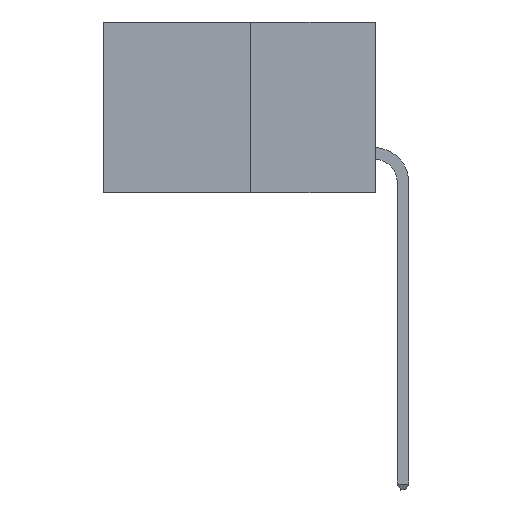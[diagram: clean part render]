
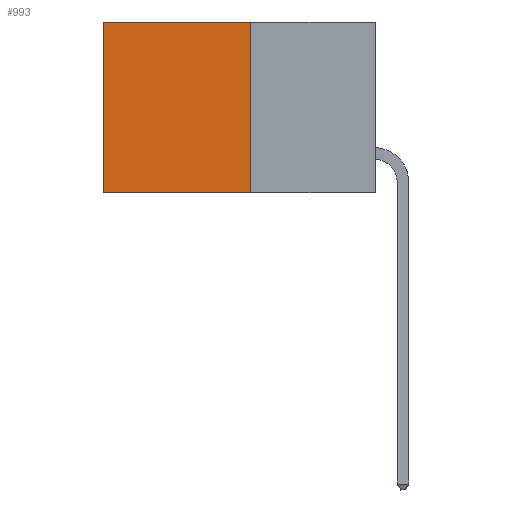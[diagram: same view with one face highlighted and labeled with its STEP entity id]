
A CAD part, left-side view. The second image highlights one B-rep face of the part: STEP entity #993.
In plain terms, the highlighted planar face has unit normal (-1, 0, 0).
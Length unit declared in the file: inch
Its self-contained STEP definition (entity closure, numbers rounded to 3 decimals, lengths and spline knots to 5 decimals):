
#87 = LINE ( 'NONE', #1131, #11337 ) ;
#577 = EDGE_CURVE ( 'NONE', #2310, #938, #10848, .T. ) ;
#585 = DIRECTION ( 'NONE',  ( 0., 1., 0. ) ) ;
#938 = VERTEX_POINT ( 'NONE', #11036 ) ;
#993 = ADVANCED_FACE ( 'NONE', ( #7029 ), #5491, .F. ) ;
#1131 = CARTESIAN_POINT ( 'NONE',  ( 0.277, 0.59, -0.37 ) ) ;
#1203 = DIRECTION ( 'NONE',  ( 0., 0., -1. ) ) ;
#1781 = VECTOR ( 'NONE', #585, 39.37008 ) ;
#2198 = VERTEX_POINT ( 'NONE', #9587 ) ;
#2310 = VERTEX_POINT ( 'NONE', #6604 ) ;
#2346 = EDGE_CURVE ( 'NONE', #10429, #2198, #8640, .T. ) ;
#3543 = VECTOR ( 'NONE', #5954, 39.37008 ) ;
#4050 = LINE ( 'NONE', #11639, #11327 ) ;
#4803 = CARTESIAN_POINT ( 'NONE',  ( 0.277, 0.27, -0.37 ) ) ;
#4816 = CARTESIAN_POINT ( 'NONE',  ( 0.277, 0.27, 0. ) ) ;
#5102 = ORIENTED_EDGE ( 'NONE', *, *, #10479, .T. ) ;
#5336 = DIRECTION ( 'NONE',  ( 0., 0., -1. ) ) ;
#5491 = PLANE ( 'NONE',  #8079 ) ;
#5525 = CARTESIAN_POINT ( 'NONE',  ( 0.277, 0.27, 0. ) ) ;
#5954 = DIRECTION ( 'NONE',  ( 0., 1., 0. ) ) ;
#5956 = EDGE_LOOP ( 'NONE', ( #5102, #6935, #9717, #8720 ) ) ;
#6604 = CARTESIAN_POINT ( 'NONE',  ( 0.277, 0.27, -0.37 ) ) ;
#6827 = DIRECTION ( 'NONE',  ( 0., 0., -1. ) ) ;
#6935 = ORIENTED_EDGE ( 'NONE', *, *, #577, .F. ) ;
#7029 = FACE_OUTER_BOUND ( 'NONE', #5956, .T. ) ;
#7379 = EDGE_CURVE ( 'NONE', #10429, #2310, #4050, .T. ) ;
#8079 = AXIS2_PLACEMENT_3D ( 'NONE', #4803, #8428, #1203 ) ;
#8428 = DIRECTION ( 'NONE',  ( 1., 0., 0. ) ) ;
#8640 = LINE ( 'NONE', #5525, #1781 ) ;
#8720 = ORIENTED_EDGE ( 'NONE', *, *, #2346, .T. ) ;
#8822 = CARTESIAN_POINT ( 'NONE',  ( 0.277, 0.27, -0.37 ) ) ;
#9587 = CARTESIAN_POINT ( 'NONE',  ( 0.277, 0.59, 0. ) ) ;
#9717 = ORIENTED_EDGE ( 'NONE', *, *, #7379, .F. ) ;
#10429 = VERTEX_POINT ( 'NONE', #4816 ) ;
#10479 = EDGE_CURVE ( 'NONE', #2198, #938, #87, .T. ) ;
#10848 = LINE ( 'NONE', #8822, #3543 ) ;
#11036 = CARTESIAN_POINT ( 'NONE',  ( 0.277, 0.59, -0.37 ) ) ;
#11327 = VECTOR ( 'NONE', #5336, 39.37008 ) ;
#11337 = VECTOR ( 'NONE', #6827, 39.37008 ) ;
#11639 = CARTESIAN_POINT ( 'NONE',  ( 0.277, 0.27, -0.37 ) ) ;
